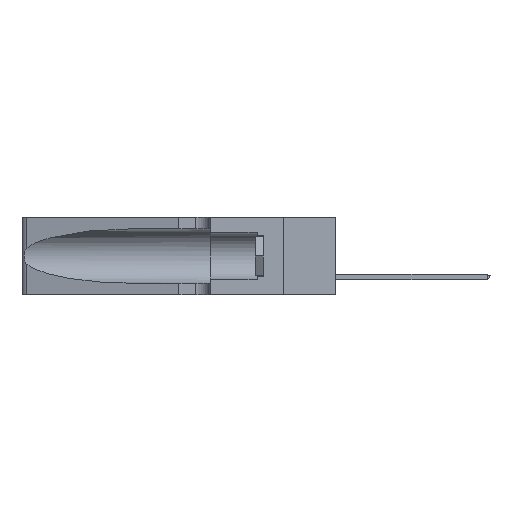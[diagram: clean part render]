
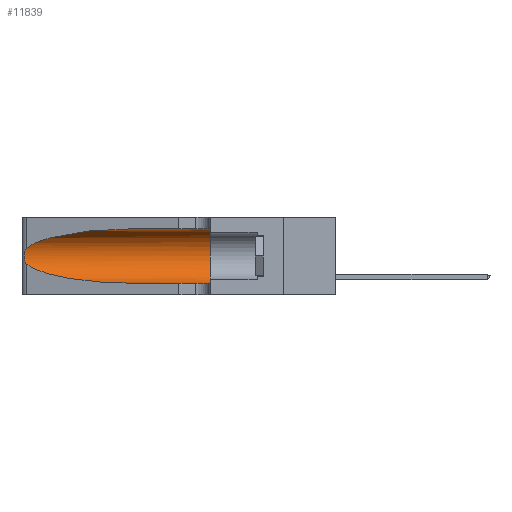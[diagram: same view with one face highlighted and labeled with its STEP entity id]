
A CAD part, left-side view. The second image highlights one B-rep face of the part: STEP entity #11839.
In plain terms, the highlighted cylindrical face has radius 3.308 mm (diameter 6.617 mm), a partial arc.
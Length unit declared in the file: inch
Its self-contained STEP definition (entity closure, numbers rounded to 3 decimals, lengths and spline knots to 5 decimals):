
#1677 = ORIENTED_EDGE ( 'NONE', *, *, #45674, .F. ) ;
#1828 = VERTEX_POINT ( 'NONE', #42421 ) ;
#1843 = CIRCLE ( 'NONE', #37834, 0.13025 ) ;
#2854 = CARTESIAN_POINT ( 'NONE',  ( 0.25555, 1.22993, 0.14849 ) ) ;
#3518 = EDGE_CURVE ( 'NONE', #41421, #23262, #11921, .T. ) ;
#3521 = CARTESIAN_POINT ( 'NONE',  ( 0.1305, 0.72297, 0.05475 ) ) ;
#4437 = CARTESIAN_POINT ( 'NONE',  ( 0.1305, 0.72297, 0.31525 ) ) ;
#4990 =( BOUNDED_CURVE ( )  B_SPLINE_CURVE ( 3, ( #29938, #42853, #50750, #3521 ),
 .UNSPECIFIED., .F., .F. ) 
 B_SPLINE_CURVE_WITH_KNOTS ( ( 4, 4 ),
 ( 3.44316, 4.71239 ),
 .UNSPECIFIED. ) 
 CURVE ( )  GEOMETRIC_REPRESENTATION_ITEM ( )  RATIONAL_B_SPLINE_CURVE ( ( 1., 0.87, 0.87, 1. ) ) 
 REPRESENTATION_ITEM ( '' )  );
#5116 = CYLINDRICAL_SURFACE ( 'NONE', #49050, 0.13025 ) ;
#5382 = CARTESIAN_POINT ( 'NONE',  ( 0.1305, 0.72297, 0.31525 ) ) ;
#6166 = DIRECTION ( 'NONE',  ( 0., -1., 0. ) ) ;
#6609 = CARTESIAN_POINT ( 'NONE',  ( 0.25555, 1.22994, 0.2215 ) ) ;
#6967 = CARTESIAN_POINT ( 'NONE',  ( 0.25787, 1.23484, 0.2124 ) ) ;
#7383 = VERTEX_POINT ( 'NONE', #21857 ) ;
#8025 = CARTESIAN_POINT ( 'NONE',  ( 0.25487, 1.22718, 0.22369 ) ) ;
#8320 = CARTESIAN_POINT ( 'NONE',  ( 0.1305, 0.35, 0.185 ) ) ;
#9667 = EDGE_CURVE ( 'NONE', #44505, #1828, #4990, .T. ) ;
#11072 = CARTESIAN_POINT ( 'NONE',  ( 0.25854, 1.2359, 0.20912 ) ) ;
#11839 = ADVANCED_FACE ( 'NONE', ( #45246 ), #5116, .F. ) ;
#11921 =( BOUNDED_CURVE ( )  B_SPLINE_CURVE ( 3, ( #4437, #24447, #19822, #8025 ),
 .UNSPECIFIED., .F., .T. ) 
 B_SPLINE_CURVE_WITH_KNOTS ( ( 4, 4 ),
 ( 1.5708, 2.84003 ),
 .UNSPECIFIED. ) 
 CURVE ( )  GEOMETRIC_REPRESENTATION_ITEM ( )  RATIONAL_B_SPLINE_CURVE ( ( 1., 0.87, 0.87, 1. ) ) 
 REPRESENTATION_ITEM ( '' )  );
#12285 = DIRECTION ( 'NONE',  ( 0., 0., 1. ) ) ;
#12456 = CARTESIAN_POINT ( 'NONE',  ( 0.25487, 1.22718, 0.22369 ) ) ;
#13671 = DIRECTION ( 'NONE',  ( 0., -1., 0. ) ) ;
#14554 = CARTESIAN_POINT ( 'NONE',  ( 0.26018, 1.23835, 0.19895 ) ) ;
#17659 = DIRECTION ( 'NONE',  ( 0., 0., -1. ) ) ;
#18950 = ORIENTED_EDGE ( 'NONE', *, *, #28404, .F. ) ;
#19059 = CARTESIAN_POINT ( 'NONE',  ( 0.26075, 1.23896, 0.178 ) ) ;
#19822 = CARTESIAN_POINT ( 'NONE',  ( 0.2373, 1.15595, 0.28018 ) ) ;
#20856 = VECTOR ( 'NONE', #35620, 39.37008 ) ;
#21849 = EDGE_CURVE ( 'NONE', #1828, #7383, #43910, .T. ) ;
#21857 = CARTESIAN_POINT ( 'NONE',  ( 0.1305, 0.35, 0.05475 ) ) ;
#22302 = VECTOR ( 'NONE', #6166, 39.37008 ) ;
#22625 = ORIENTED_EDGE ( 'NONE', *, *, #9667, .T. ) ;
#23262 = VERTEX_POINT ( 'NONE', #12456 ) ;
#24447 = CARTESIAN_POINT ( 'NONE',  ( 0.18966, 0.96281, 0.31525 ) ) ;
#24571 = LINE ( 'NONE', #27327, #20856 ) ;
#26457 = CARTESIAN_POINT ( 'NONE',  ( 0.25856, 1.23593, 0.16098 ) ) ;
#27327 = CARTESIAN_POINT ( 'NONE',  ( 0.1305, 1.61858, 0.31525 ) ) ;
#28138 = VERTEX_POINT ( 'NONE', #41601 ) ;
#28404 = EDGE_CURVE ( 'NONE', #41421, #28138, #24571, .T. ) ;
#29186 = EDGE_CURVE ( 'NONE', #23262, #44505, #30377, .T. ) ;
#29938 = CARTESIAN_POINT ( 'NONE',  ( 0.25487, 1.22718, 0.14631 ) ) ;
#30144 = CARTESIAN_POINT ( 'NONE',  ( 0.25789, 1.23486, 0.15765 ) ) ;
#30377 = B_SPLINE_CURVE_WITH_KNOTS ( 'NONE', 3,
 ( #30673, #6609, #42676, #6967, #11072, #14554, #50084, #19059, #49741, #26457, #30144, #34089, #2854, #30500 ),
 .UNSPECIFIED., .F., .F.,
 ( 4, 2, 2, 2, 2, 2, 4 ),
 ( 0., 0.00027, 0.00053, 0.00107, 0.0016, 0.00187, 0.00214 ),
 .UNSPECIFIED. ) ;
#30500 = CARTESIAN_POINT ( 'NONE',  ( 0.25487, 1.22718, 0.14631 ) ) ;
#30673 = CARTESIAN_POINT ( 'NONE',  ( 0.25487, 1.22718, 0.22369 ) ) ;
#33383 = ORIENTED_EDGE ( 'NONE', *, *, #21849, .T. ) ;
#33646 = ORIENTED_EDGE ( 'NONE', *, *, #29186, .T. ) ;
#34089 = CARTESIAN_POINT ( 'NONE',  ( 0.25639, 1.23186, 0.15144 ) ) ;
#34185 = CARTESIAN_POINT ( 'NONE',  ( 0.1305, 1.61858, 0.05475 ) ) ;
#35567 = CARTESIAN_POINT ( 'NONE',  ( 0.25487, 1.22718, 0.14631 ) ) ;
#35620 = DIRECTION ( 'NONE',  ( 0., -1., 0. ) ) ;
#37337 = CARTESIAN_POINT ( 'NONE',  ( 0.1305, 1.61858, 0.185 ) ) ;
#37834 = AXIS2_PLACEMENT_3D ( 'NONE', #8320, #39968, #12285 ) ;
#39968 = DIRECTION ( 'NONE',  ( 0., 1., 0. ) ) ;
#41421 = VERTEX_POINT ( 'NONE', #5382 ) ;
#41601 = CARTESIAN_POINT ( 'NONE',  ( 0.1305, 0.35, 0.31525 ) ) ;
#41951 = ORIENTED_EDGE ( 'NONE', *, *, #3518, .T. ) ;
#42421 = CARTESIAN_POINT ( 'NONE',  ( 0.1305, 0.72297, 0.05475 ) ) ;
#42676 = CARTESIAN_POINT ( 'NONE',  ( 0.25639, 1.23184, 0.21858 ) ) ;
#42853 = CARTESIAN_POINT ( 'NONE',  ( 0.2373, 1.15595, 0.08982 ) ) ;
#43358 = EDGE_LOOP ( 'NONE', ( #41951, #33646, #22625, #33383, #1677, #18950 ) ) ;
#43910 = LINE ( 'NONE', #34185, #22302 ) ;
#44505 = VERTEX_POINT ( 'NONE', #35567 ) ;
#45246 = FACE_OUTER_BOUND ( 'NONE', #43358, .T. ) ;
#45674 = EDGE_CURVE ( 'NONE', #28138, #7383, #1843, .T. ) ;
#49050 = AXIS2_PLACEMENT_3D ( 'NONE', #37337, #13671, #17659 ) ;
#49741 = CARTESIAN_POINT ( 'NONE',  ( 0.26017, 1.23833, 0.17102 ) ) ;
#50084 = CARTESIAN_POINT ( 'NONE',  ( 0.26075, 1.23896, 0.19203 ) ) ;
#50750 = CARTESIAN_POINT ( 'NONE',  ( 0.18966, 0.96281, 0.05475 ) ) ;
